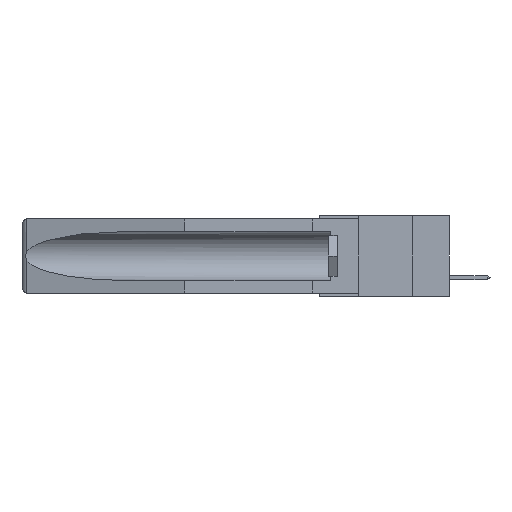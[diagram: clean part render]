
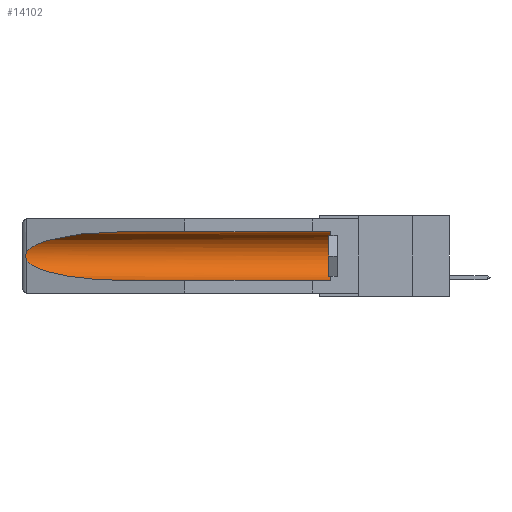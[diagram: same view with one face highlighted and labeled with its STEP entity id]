
A CAD part, left-side view. The second image highlights one B-rep face of the part: STEP entity #14102.
In plain terms, the highlighted cylindrical face has radius 2.857 mm (diameter 5.715 mm), a partial arc.
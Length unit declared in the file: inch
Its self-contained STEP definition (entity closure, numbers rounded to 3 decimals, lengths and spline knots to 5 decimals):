
#92 = FACE_OUTER_BOUND ( 'NONE', #9368, .T. ) ;
#1031 = CARTESIAN_POINT ( 'NONE',  ( 0.26597, 1.52961, -0.15275 ) ) ;
#1949 = AXIS2_PLACEMENT_3D ( 'NONE', #14623, #10304, #11736 ) ;
#2123 = VERTEX_POINT ( 'NONE', #3885 ) ;
#2256 = ORIENTED_EDGE ( 'NONE', *, *, #3041, .T. ) ;
#2261 = EDGE_CURVE ( 'NONE', #2123, #12117, #4781, .T. ) ;
#2383 =( BOUNDED_CURVE ( )  B_SPLINE_CURVE ( 3, ( #2539, #12560, #5401, #18192 ),
 .UNSPECIFIED., .F., .F. ) 
 B_SPLINE_CURVE_WITH_KNOTS ( ( 4, 4 ),
 ( 0.1948, 1.5708 ),
 .UNSPECIFIED. ) 
 CURVE ( )  GEOMETRIC_REPRESENTATION_ITEM ( )  RATIONAL_B_SPLINE_CURVE ( ( 1., 0.848, 0.848, 1. ) ) 
 REPRESENTATION_ITEM ( '' )  );
#2539 = CARTESIAN_POINT ( 'NONE',  ( 0.26537, 1.52718, -0.19328 ) ) ;
#3041 = EDGE_CURVE ( 'NONE', #13191, #18227, #6245, .T. ) ;
#3277 = ORIENTED_EDGE ( 'NONE', *, *, #7814, .T. ) ;
#3426 = DIRECTION ( 'NONE',  ( 0., 1., 0. ) ) ;
#3885 = CARTESIAN_POINT ( 'NONE',  ( 0.26537, 1.52718, -0.14972 ) ) ;
#3960 = CARTESIAN_POINT ( 'NONE',  ( 0.26655, 1.53094, -0.18657 ) ) ;
#4031 = ORIENTED_EDGE ( 'NONE', *, *, #14904, .F. ) ;
#4781 = B_SPLINE_CURVE_WITH_KNOTS ( 'NONE', 3,
 ( #6688, #1031, #11057, #12486, #8037, #10993, #12539, #3960, #15122, #16820 ),
 .UNSPECIFIED., .F., .F.,
 ( 4, 2, 2, 2, 4 ),
 ( 0., 0.00029, 0.00058, 0.00087, 0.00117 ),
 .UNSPECIFIED. ) ;
#4797 = CARTESIAN_POINT ( 'NONE',  ( 0.25451, 1.48313, -0.09465 ) ) ;
#5045 = DIRECTION ( 'NONE',  ( 0., 0., 1. ) ) ;
#5294 = AXIS2_PLACEMENT_3D ( 'NONE', #12138, #15029, #5045 ) ;
#5401 = CARTESIAN_POINT ( 'NONE',  ( 0.21114, 1.30732, -0.284 ) ) ;
#6136 = ORIENTED_EDGE ( 'NONE', *, *, #10915, .T. ) ;
#6245 = CIRCLE ( 'NONE', #5294, 0.1125 ) ;
#6688 = CARTESIAN_POINT ( 'NONE',  ( 0.26537, 1.52718, -0.14972 ) ) ;
#6777 =( BOUNDED_CURVE ( )  B_SPLINE_CURVE ( 3, ( #10464, #13400, #4797, #14834 ),
 .UNSPECIFIED., .F., .F. ) 
 B_SPLINE_CURVE_WITH_KNOTS ( ( 4, 4 ),
 ( 4.71239, 6.08839 ),
 .UNSPECIFIED. ) 
 CURVE ( )  GEOMETRIC_REPRESENTATION_ITEM ( )  RATIONAL_B_SPLINE_CURVE ( ( 1., 0.848, 0.848, 1. ) ) 
 REPRESENTATION_ITEM ( '' )  );
#6839 = VERTEX_POINT ( 'NONE', #15130 ) ;
#6865 = CARTESIAN_POINT ( 'NONE',  ( 0.155, 0.126, -0.284 ) ) ;
#7136 = VECTOR ( 'NONE', #14941, 39.37008 ) ;
#7814 = EDGE_CURVE ( 'NONE', #6839, #2123, #6777, .T. ) ;
#7889 = VECTOR ( 'NONE', #3426, 39.37008 ) ;
#8025 = CARTESIAN_POINT ( 'NONE',  ( 0.26537, 1.52718, -0.19328 ) ) ;
#8037 = CARTESIAN_POINT ( 'NONE',  ( 0.2675, 1.53308, -0.16763 ) ) ;
#8058 = VERTEX_POINT ( 'NONE', #12564 ) ;
#8255 = ORIENTED_EDGE ( 'NONE', *, *, #10511, .T. ) ;
#8810 = CARTESIAN_POINT ( 'NONE',  ( 0.155, 0.126, -0.059 ) ) ;
#9368 = EDGE_LOOP ( 'NONE', ( #3277, #16236, #8255, #4031, #2256, #6136 ) ) ;
#10304 = DIRECTION ( 'NONE',  ( 0., 1., 0. ) ) ;
#10464 = CARTESIAN_POINT ( 'NONE',  ( 0.155, 1.07973, -0.059 ) ) ;
#10511 = EDGE_CURVE ( 'NONE', #12117, #8058, #2383, .T. ) ;
#10779 = CARTESIAN_POINT ( 'NONE',  ( 0.155, -0.30754, -0.284 ) ) ;
#10830 = CYLINDRICAL_SURFACE ( 'NONE', #1949, 0.1125 ) ;
#10915 = EDGE_CURVE ( 'NONE', #18227, #6839, #12315, .T. ) ;
#10993 = CARTESIAN_POINT ( 'NONE',  ( 0.2675, 1.53308, -0.17534 ) ) ;
#11057 = CARTESIAN_POINT ( 'NONE',  ( 0.26654, 1.53092, -0.15636 ) ) ;
#11736 = DIRECTION ( 'NONE',  ( 0., 0., 1. ) ) ;
#11995 = CARTESIAN_POINT ( 'NONE',  ( 0.155, -0.30754, -0.059 ) ) ;
#12117 = VERTEX_POINT ( 'NONE', #8025 ) ;
#12138 = CARTESIAN_POINT ( 'NONE',  ( 0.155, 0.126, -0.1715 ) ) ;
#12315 = LINE ( 'NONE', #11995, #7136 ) ;
#12486 = CARTESIAN_POINT ( 'NONE',  ( 0.2673, 1.5327, -0.16383 ) ) ;
#12539 = CARTESIAN_POINT ( 'NONE',  ( 0.2673, 1.53269, -0.17917 ) ) ;
#12560 = CARTESIAN_POINT ( 'NONE',  ( 0.25451, 1.48313, -0.24835 ) ) ;
#12564 = CARTESIAN_POINT ( 'NONE',  ( 0.155, 1.07973, -0.284 ) ) ;
#13191 = VERTEX_POINT ( 'NONE', #6865 ) ;
#13400 = CARTESIAN_POINT ( 'NONE',  ( 0.21114, 1.30732, -0.059 ) ) ;
#14102 = ADVANCED_FACE ( 'NONE', ( #92 ), #10830, .F. ) ;
#14623 = CARTESIAN_POINT ( 'NONE',  ( 0.155, -0.30754, -0.1715 ) ) ;
#14834 = CARTESIAN_POINT ( 'NONE',  ( 0.26537, 1.52718, -0.14972 ) ) ;
#14847 = LINE ( 'NONE', #10779, #7889 ) ;
#14904 = EDGE_CURVE ( 'NONE', #13191, #8058, #14847, .T. ) ;
#14941 = DIRECTION ( 'NONE',  ( 0., 1., 0. ) ) ;
#15029 = DIRECTION ( 'NONE',  ( 0., -1., 0. ) ) ;
#15122 = CARTESIAN_POINT ( 'NONE',  ( 0.26597, 1.5296, -0.19026 ) ) ;
#15130 = CARTESIAN_POINT ( 'NONE',  ( 0.155, 1.07973, -0.059 ) ) ;
#16236 = ORIENTED_EDGE ( 'NONE', *, *, #2261, .T. ) ;
#16820 = CARTESIAN_POINT ( 'NONE',  ( 0.26537, 1.52718, -0.19328 ) ) ;
#18192 = CARTESIAN_POINT ( 'NONE',  ( 0.155, 1.07973, -0.284 ) ) ;
#18227 = VERTEX_POINT ( 'NONE', #8810 ) ;
